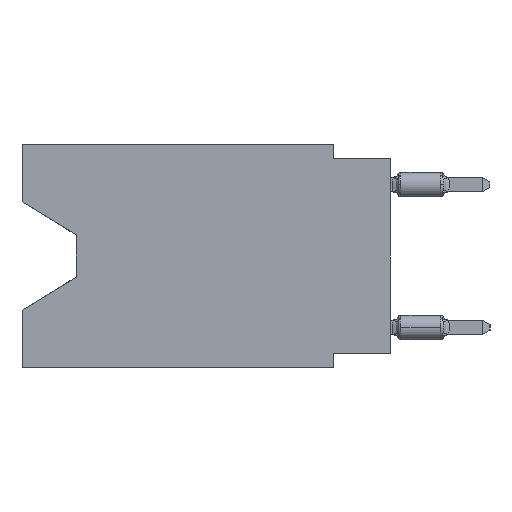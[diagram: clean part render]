
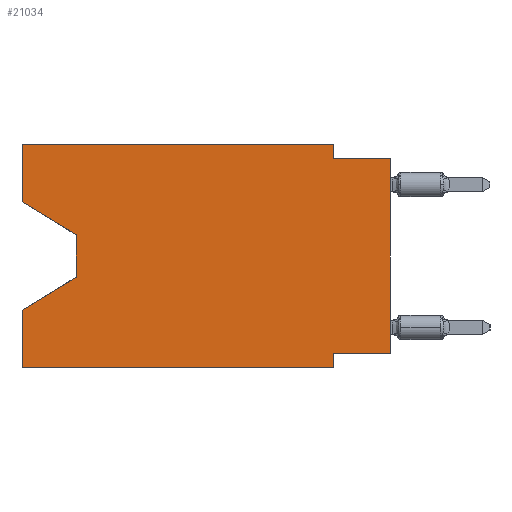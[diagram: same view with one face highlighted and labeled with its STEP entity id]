
A CAD part, left-side view. The second image highlights one B-rep face of the part: STEP entity #21034.
In plain terms, the highlighted planar face has unit normal (-1, 0, 0).
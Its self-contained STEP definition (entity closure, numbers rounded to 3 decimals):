
#132 = CARTESIAN_POINT ( 'NONE',  ( 0., 16.383, -9.906 ) ) ;
#1038 = CARTESIAN_POINT ( 'NONE',  ( 0., 2.54, -0.635 ) ) ;
#1474 = CARTESIAN_POINT ( 'NONE',  ( 0., 16.383, 0. ) ) ;
#1545 = VERTEX_POINT ( 'NONE', #15421 ) ;
#1961 = DIRECTION ( 'NONE',  ( 0., -1., 0. ) ) ;
#2483 = ORIENTED_EDGE ( 'NONE', *, *, #3884, .F. ) ;
#2749 = PLANE ( 'NONE',  #14027 ) ;
#2917 = LINE ( 'NONE', #23348, #9483 ) ;
#3084 = VECTOR ( 'NONE', #3616, 1000. ) ;
#3256 = LINE ( 'NONE', #16470, #3084 ) ;
#3555 = LINE ( 'NONE', #11025, #12670 ) ;
#3616 = DIRECTION ( 'NONE',  ( 0., -0.855, -0.519 ) ) ;
#3884 = EDGE_CURVE ( 'NONE', #20296, #19647, #9203, .T. ) ;
#4202 = CARTESIAN_POINT ( 'NONE',  ( 0., 0., -9.271 ) ) ;
#4322 = DIRECTION ( 'NONE',  ( 0., 0., -1. ) ) ;
#4568 = EDGE_CURVE ( 'NONE', #21010, #8275, #2917, .T. ) ;
#5119 = CARTESIAN_POINT ( 'NONE',  ( 0., 16.383, 0. ) ) ;
#5757 = EDGE_CURVE ( 'NONE', #1545, #14012, #17517, .T. ) ;
#5833 = VERTEX_POINT ( 'NONE', #8115 ) ;
#5856 = CARTESIAN_POINT ( 'NONE',  ( 0., 13.97, -4.013 ) ) ;
#5922 = VERTEX_POINT ( 'NONE', #5856 ) ;
#6311 = ORIENTED_EDGE ( 'NONE', *, *, #15769, .T. ) ;
#7045 = ORIENTED_EDGE ( 'NONE', *, *, #20755, .T. ) ;
#7108 = DIRECTION ( 'NONE',  ( 0., 0., -1. ) ) ;
#7161 = VECTOR ( 'NONE', #23029, 1000. ) ;
#7190 = EDGE_CURVE ( 'NONE', #9444, #14550, #3555, .T. ) ;
#7608 = DIRECTION ( 'NONE',  ( 0., -1., 0. ) ) ;
#7999 = EDGE_CURVE ( 'NONE', #19647, #21010, #14859, .T. ) ;
#8056 = CARTESIAN_POINT ( 'NONE',  ( 0., 2.54, -9.906 ) ) ;
#8115 = CARTESIAN_POINT ( 'NONE',  ( 0., 0., -9.271 ) ) ;
#8275 = VERTEX_POINT ( 'NONE', #10552 ) ;
#8330 = ORIENTED_EDGE ( 'NONE', *, *, #7999, .F. ) ;
#8514 = ORIENTED_EDGE ( 'NONE', *, *, #7190, .F. ) ;
#9016 = CARTESIAN_POINT ( 'NONE',  ( 0., 16.383, 0. ) ) ;
#9080 = DIRECTION ( 'NONE',  ( 0., 0., 1. ) ) ;
#9203 = LINE ( 'NONE', #11264, #11900 ) ;
#9444 = VERTEX_POINT ( 'NONE', #10713 ) ;
#9483 = VECTOR ( 'NONE', #21857, 1000. ) ;
#10215 = CARTESIAN_POINT ( 'NONE',  ( 0., 16.383, 0. ) ) ;
#10552 = CARTESIAN_POINT ( 'NONE',  ( 0., 0., -0.635 ) ) ;
#10652 = LINE ( 'NONE', #1474, #21848 ) ;
#10713 = CARTESIAN_POINT ( 'NONE',  ( 0., 2.54, -9.271 ) ) ;
#10735 = LINE ( 'NONE', #23828, #13723 ) ;
#10851 = EDGE_CURVE ( 'NONE', #22123, #14012, #13169, .T. ) ;
#11025 = CARTESIAN_POINT ( 'NONE',  ( 0., 2.54, -9.906 ) ) ;
#11137 = CARTESIAN_POINT ( 'NONE',  ( 0., 16.383, -7.36 ) ) ;
#11264 = CARTESIAN_POINT ( 'NONE',  ( 0., 16.383, 0. ) ) ;
#11299 = LINE ( 'NONE', #4202, #14538 ) ;
#11690 = ORIENTED_EDGE ( 'NONE', *, *, #4568, .F. ) ;
#11900 = VECTOR ( 'NONE', #1961, 1000. ) ;
#12180 = VECTOR ( 'NONE', #20746, 1000. ) ;
#12270 = ORIENTED_EDGE ( 'NONE', *, *, #5757, .T. ) ;
#12314 = VERTEX_POINT ( 'NONE', #16925 ) ;
#12555 = ORIENTED_EDGE ( 'NONE', *, *, #17724, .F. ) ;
#12670 = VECTOR ( 'NONE', #7108, 1000. ) ;
#12918 = ORIENTED_EDGE ( 'NONE', *, *, #17096, .T. ) ;
#13118 = EDGE_CURVE ( 'NONE', #5922, #1545, #10735, .T. ) ;
#13169 = LINE ( 'NONE', #9016, #12180 ) ;
#13723 = VECTOR ( 'NONE', #16609, 1000. ) ;
#13766 = DIRECTION ( 'NONE',  ( 1., 0., 0. ) ) ;
#14012 = VERTEX_POINT ( 'NONE', #11137 ) ;
#14027 = AXIS2_PLACEMENT_3D ( 'NONE', #10215, #13766, #21223 ) ;
#14538 = VECTOR ( 'NONE', #16812, 1000. ) ;
#14550 = VERTEX_POINT ( 'NONE', #8056 ) ;
#14859 = LINE ( 'NONE', #23041, #16606 ) ;
#14917 = ORIENTED_EDGE ( 'NONE', *, *, #18136, .F. ) ;
#15421 = CARTESIAN_POINT ( 'NONE',  ( 0., 13.97, -5.893 ) ) ;
#15769 = EDGE_CURVE ( 'NONE', #5833, #8275, #18610, .T. ) ;
#16028 = CARTESIAN_POINT ( 'NONE',  ( 0., 2.54, 0. ) ) ;
#16470 = CARTESIAN_POINT ( 'NONE',  ( 0., 16.383, -2.546 ) ) ;
#16606 = VECTOR ( 'NONE', #4322, 1000. ) ;
#16609 = DIRECTION ( 'NONE',  ( 0., 0., -1. ) ) ;
#16812 = DIRECTION ( 'NONE',  ( 0., 1., 0. ) ) ;
#16904 = CARTESIAN_POINT ( 'NONE',  ( 0., 0., 0. ) ) ;
#16925 = CARTESIAN_POINT ( 'NONE',  ( 0., 16.383, -2.546 ) ) ;
#17096 = EDGE_CURVE ( 'NONE', #22123, #14550, #18609, .T. ) ;
#17485 = ORIENTED_EDGE ( 'NONE', *, *, #10851, .F. ) ;
#17517 = LINE ( 'NONE', #20157, #7161 ) ;
#17724 = EDGE_CURVE ( 'NONE', #5833, #9444, #11299, .T. ) ;
#17942 = ORIENTED_EDGE ( 'NONE', *, *, #13118, .T. ) ;
#18074 = EDGE_LOOP ( 'NONE', ( #7045, #17942, #12270, #17485, #12918, #8514, #12555, #6311, #11690, #8330, #2483, #14917 ) ) ;
#18136 = EDGE_CURVE ( 'NONE', #12314, #20296, #10652, .T. ) ;
#18609 = LINE ( 'NONE', #132, #24012 ) ;
#18610 = LINE ( 'NONE', #16904, #22005 ) ;
#18728 = DIRECTION ( 'NONE',  ( 0., 0., 1. ) ) ;
#19044 = CARTESIAN_POINT ( 'NONE',  ( 0., 16.383, -9.906 ) ) ;
#19647 = VERTEX_POINT ( 'NONE', #16028 ) ;
#20157 = CARTESIAN_POINT ( 'NONE',  ( 0., 13.97, -5.893 ) ) ;
#20296 = VERTEX_POINT ( 'NONE', #5119 ) ;
#20746 = DIRECTION ( 'NONE',  ( 0., 0., 1. ) ) ;
#20755 = EDGE_CURVE ( 'NONE', #12314, #5922, #3256, .T. ) ;
#21010 = VERTEX_POINT ( 'NONE', #1038 ) ;
#21034 = ADVANCED_FACE ( 'NONE', ( #21102 ), #2749, .F. ) ;
#21102 = FACE_OUTER_BOUND ( 'NONE', #18074, .T. ) ;
#21223 = DIRECTION ( 'NONE',  ( 0., 0., -1. ) ) ;
#21848 = VECTOR ( 'NONE', #9080, 1000. ) ;
#21857 = DIRECTION ( 'NONE',  ( 0., -1., 0. ) ) ;
#22005 = VECTOR ( 'NONE', #18728, 1000. ) ;
#22123 = VERTEX_POINT ( 'NONE', #19044 ) ;
#23029 = DIRECTION ( 'NONE',  ( 0., 0.855, -0.519 ) ) ;
#23041 = CARTESIAN_POINT ( 'NONE',  ( 0., 2.54, 0. ) ) ;
#23348 = CARTESIAN_POINT ( 'NONE',  ( 0., 0., -0.635 ) ) ;
#23828 = CARTESIAN_POINT ( 'NONE',  ( 0., 13.97, -4.013 ) ) ;
#24012 = VECTOR ( 'NONE', #7608, 1000. ) ;
